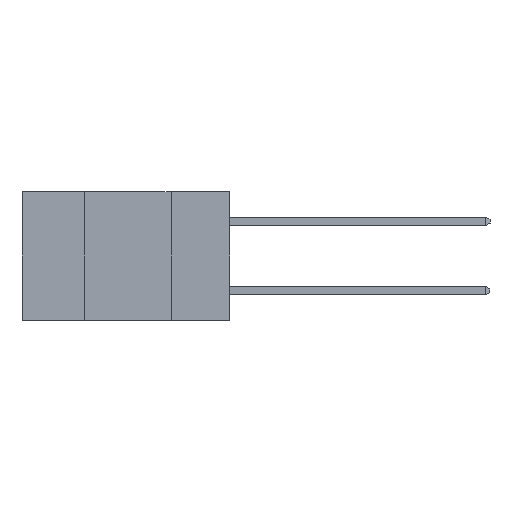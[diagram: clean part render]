
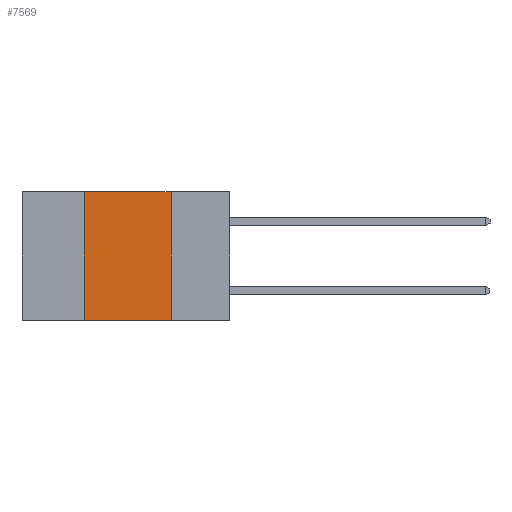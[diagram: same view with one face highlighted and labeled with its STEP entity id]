
A CAD part, left-side view. The second image highlights one B-rep face of the part: STEP entity #7569.
In plain terms, the highlighted planar face has unit normal (-1, 0, 0).
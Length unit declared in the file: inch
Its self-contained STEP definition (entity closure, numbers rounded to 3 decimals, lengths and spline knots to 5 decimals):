
#33 = VECTOR ( 'NONE', #15089, 39.37008 ) ;
#279 = LINE ( 'NONE', #2151, #6124 ) ;
#354 = VERTEX_POINT ( 'NONE', #6665 ) ;
#651 = CARTESIAN_POINT ( 'NONE',  ( 0., 0.17, 0. ) ) ;
#1148 = DIRECTION ( 'NONE',  ( 1., 0., 0. ) ) ;
#2151 = CARTESIAN_POINT ( 'NONE',  ( 0., 0.17, 0. ) ) ;
#3415 = CARTESIAN_POINT ( 'NONE',  ( 0., 0.6, 0. ) ) ;
#4019 = CARTESIAN_POINT ( 'NONE',  ( 0., 0.42, 0. ) ) ;
#4566 = ORIENTED_EDGE ( 'NONE', *, *, #9644, .F. ) ;
#4599 = DIRECTION ( 'NONE',  ( 0., -1., 0. ) ) ;
#4836 = LINE ( 'NONE', #6352, #11472 ) ;
#6124 = VECTOR ( 'NONE', #9253, 39.37008 ) ;
#6189 = EDGE_CURVE ( 'NONE', #354, #13336, #12486, .T. ) ;
#6352 = CARTESIAN_POINT ( 'NONE',  ( 0., 0.6, -0.37 ) ) ;
#6665 = CARTESIAN_POINT ( 'NONE',  ( 0., 0.42, -0.37 ) ) ;
#7569 = ADVANCED_FACE ( 'NONE', ( #8600 ), #15190, .F. ) ;
#8176 = ORIENTED_EDGE ( 'NONE', *, *, #6189, .F. ) ;
#8353 = VECTOR ( 'NONE', #4599, 39.37008 ) ;
#8559 = EDGE_LOOP ( 'NONE', ( #4566, #12296, #8176, #10230 ) ) ;
#8600 = FACE_OUTER_BOUND ( 'NONE', #8559, .T. ) ;
#9016 = EDGE_CURVE ( 'NONE', #13336, #14087, #14605, .T. ) ;
#9253 = DIRECTION ( 'NONE',  ( 0., 0., -1. ) ) ;
#9369 = DIRECTION ( 'NONE',  ( 0., 0., -1. ) ) ;
#9644 = EDGE_CURVE ( 'NONE', #14087, #9653, #279, .T. ) ;
#9653 = VERTEX_POINT ( 'NONE', #11591 ) ;
#9855 = DIRECTION ( 'NONE',  ( 0., -1., 0. ) ) ;
#10230 = ORIENTED_EDGE ( 'NONE', *, *, #13288, .T. ) ;
#11472 = VECTOR ( 'NONE', #9855, 39.37008 ) ;
#11591 = CARTESIAN_POINT ( 'NONE',  ( 0., 0.17, -0.37 ) ) ;
#12296 = ORIENTED_EDGE ( 'NONE', *, *, #9016, .F. ) ;
#12486 = LINE ( 'NONE', #12720, #33 ) ;
#12720 = CARTESIAN_POINT ( 'NONE',  ( 0., 0.42, 0. ) ) ;
#12841 = CARTESIAN_POINT ( 'NONE',  ( 0., 0.6, 0. ) ) ;
#13288 = EDGE_CURVE ( 'NONE', #354, #9653, #4836, .T. ) ;
#13336 = VERTEX_POINT ( 'NONE', #4019 ) ;
#13923 = AXIS2_PLACEMENT_3D ( 'NONE', #12841, #1148, #9369 ) ;
#14087 = VERTEX_POINT ( 'NONE', #651 ) ;
#14605 = LINE ( 'NONE', #3415, #8353 ) ;
#15089 = DIRECTION ( 'NONE',  ( 0., 0., 1. ) ) ;
#15190 = PLANE ( 'NONE',  #13923 ) ;
